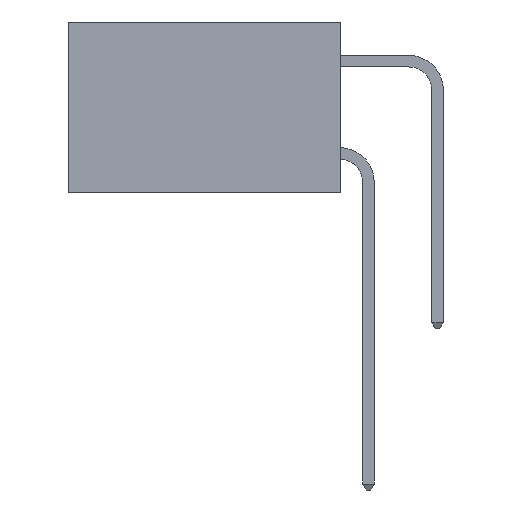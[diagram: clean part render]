
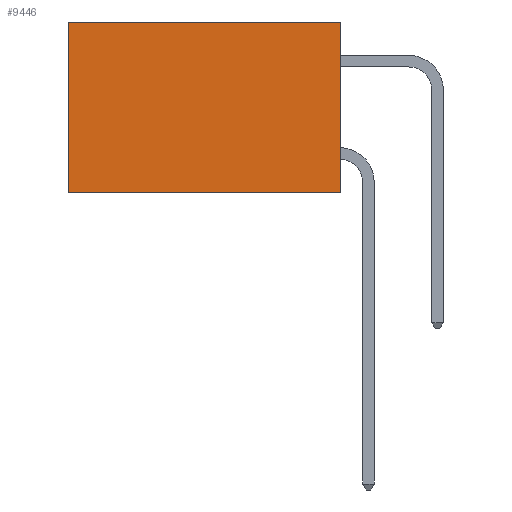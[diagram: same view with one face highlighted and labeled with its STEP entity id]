
A CAD part, left-side view. The second image highlights one B-rep face of the part: STEP entity #9446.
In plain terms, the highlighted planar face has unit normal (-1, 0, 0).
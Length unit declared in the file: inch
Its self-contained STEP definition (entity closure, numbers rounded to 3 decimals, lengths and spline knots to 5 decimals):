
#142 = VECTOR ( 'NONE', #7640, 39.37008 ) ;
#228 = VERTEX_POINT ( 'NONE', #5975 ) ;
#713 = AXIS2_PLACEMENT_3D ( 'NONE', #1357, #2645, #11476 ) ;
#1231 = EDGE_CURVE ( 'NONE', #228, #7836, #3501, .T. ) ;
#1357 = CARTESIAN_POINT ( 'NONE',  ( 0.277, 0., -0.37 ) ) ;
#2100 = EDGE_CURVE ( 'NONE', #2986, #7836, #6931, .T. ) ;
#2201 = ORIENTED_EDGE ( 'NONE', *, *, #1231, .F. ) ;
#2645 = DIRECTION ( 'NONE',  ( 1., 0., 0. ) ) ;
#2986 = VERTEX_POINT ( 'NONE', #9764 ) ;
#3248 = VECTOR ( 'NONE', #9004, 39.37008 ) ;
#3501 = LINE ( 'NONE', #10514, #142 ) ;
#4084 = CARTESIAN_POINT ( 'NONE',  ( 0.277, 0., 0. ) ) ;
#4622 = EDGE_CURVE ( 'NONE', #12983, #228, #13847, .T. ) ;
#5562 = ORIENTED_EDGE ( 'NONE', *, *, #4622, .F. ) ;
#5951 = EDGE_CURVE ( 'NONE', #12983, #2986, #10026, .T. ) ;
#5975 = CARTESIAN_POINT ( 'NONE',  ( 0.277, 0., -0.37 ) ) ;
#6253 = FACE_OUTER_BOUND ( 'NONE', #15854, .T. ) ;
#6931 = LINE ( 'NONE', #13976, #13444 ) ;
#7358 = ORIENTED_EDGE ( 'NONE', *, *, #2100, .T. ) ;
#7640 = DIRECTION ( 'NONE',  ( 0., 1., 0. ) ) ;
#7836 = VERTEX_POINT ( 'NONE', #14437 ) ;
#7941 = CARTESIAN_POINT ( 'NONE',  ( 0.277, 0., 0. ) ) ;
#8471 = DIRECTION ( 'NONE',  ( 0., 0., -1. ) ) ;
#8552 = CARTESIAN_POINT ( 'NONE',  ( 0.277, 0., -0.37 ) ) ;
#8981 = PLANE ( 'NONE',  #713 ) ;
#9004 = DIRECTION ( 'NONE',  ( 0., 1., 0. ) ) ;
#9446 = ADVANCED_FACE ( 'NONE', ( #6253 ), #8981, .F. ) ;
#9764 = CARTESIAN_POINT ( 'NONE',  ( 0.277, 0.59, 0. ) ) ;
#10026 = LINE ( 'NONE', #7941, #3248 ) ;
#10514 = CARTESIAN_POINT ( 'NONE',  ( 0.277, 0., -0.37 ) ) ;
#11019 = VECTOR ( 'NONE', #8471, 39.37008 ) ;
#11476 = DIRECTION ( 'NONE',  ( 0., 0., -1. ) ) ;
#12983 = VERTEX_POINT ( 'NONE', #4084 ) ;
#13193 = ORIENTED_EDGE ( 'NONE', *, *, #5951, .T. ) ;
#13444 = VECTOR ( 'NONE', #13974, 39.37008 ) ;
#13847 = LINE ( 'NONE', #8552, #11019 ) ;
#13974 = DIRECTION ( 'NONE',  ( 0., 0., -1. ) ) ;
#13976 = CARTESIAN_POINT ( 'NONE',  ( 0.277, 0.59, -0.37 ) ) ;
#14437 = CARTESIAN_POINT ( 'NONE',  ( 0.277, 0.59, -0.37 ) ) ;
#15854 = EDGE_LOOP ( 'NONE', ( #7358, #2201, #5562, #13193 ) ) ;
